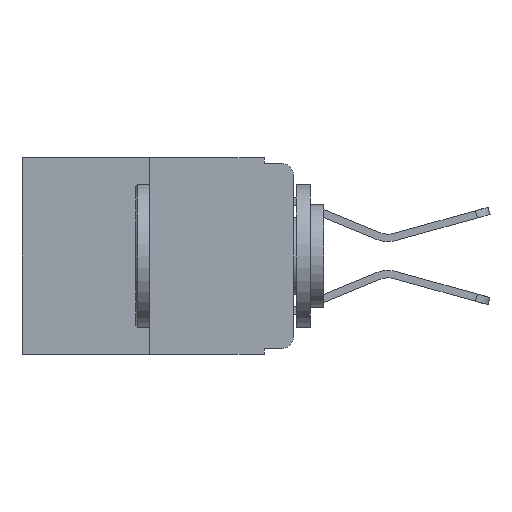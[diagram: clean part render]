
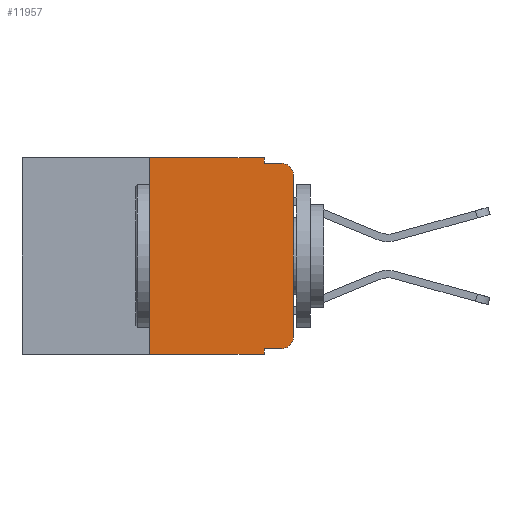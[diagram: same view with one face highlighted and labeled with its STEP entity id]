
A CAD part, left-side view. The second image highlights one B-rep face of the part: STEP entity #11957.
In plain terms, the highlighted planar face has unit normal (-1, 0, 0).
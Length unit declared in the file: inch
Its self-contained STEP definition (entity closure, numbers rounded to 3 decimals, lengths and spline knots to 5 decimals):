
#31 = CARTESIAN_POINT ( 'NONE',  ( 0., 0.051, 0. ) ) ;
#358 = DIRECTION ( 'NONE',  ( 0., 0., 1. ) ) ;
#479 = EDGE_CURVE ( 'NONE', #14245, #7207, #16732, .T. ) ;
#652 = CARTESIAN_POINT ( 'NONE',  ( 0., 0.473, 0. ) ) ;
#1036 = ORIENTED_EDGE ( 'NONE', *, *, #11001, .T. ) ;
#1067 = LINE ( 'NONE', #2929, #14947 ) ;
#1095 = VECTOR ( 'NONE', #3181, 39.37008 ) ;
#1126 = CARTESIAN_POINT ( 'NONE',  ( 0., 0.051, -0.333 ) ) ;
#1220 = DIRECTION ( 'NONE',  ( 0., 0., -1. ) ) ;
#1286 = EDGE_LOOP ( 'NONE', ( #9746, #17314, #14010, #10671, #15357, #8605, #1036, #13803, #14246, #10911 ) ) ;
#1747 = EDGE_CURVE ( 'NONE', #14640, #16593, #3908, .T. ) ;
#1892 = DIRECTION ( 'NONE',  ( 0., -1., 0. ) ) ;
#2015 = VECTOR ( 'NONE', #358, 39.37008 ) ;
#2631 = DIRECTION ( 'NONE',  ( 0., -1., 0. ) ) ;
#2929 = CARTESIAN_POINT ( 'NONE',  ( 0., 0.051, -0.01 ) ) ;
#3027 = CARTESIAN_POINT ( 'NONE',  ( 0., 0.02, -0.03 ) ) ;
#3181 = DIRECTION ( 'NONE',  ( 0., 0., -1. ) ) ;
#3718 = PLANE ( 'NONE',  #17920 ) ;
#3908 = LINE ( 'NONE', #16813, #15165 ) ;
#4431 = AXIS2_PLACEMENT_3D ( 'NONE', #6368, #7781, #1220 ) ;
#4578 = DIRECTION ( 'NONE',  ( 0., 0., -1. ) ) ;
#4724 = DIRECTION ( 'NONE',  ( 0., 0., 1. ) ) ;
#5534 = CARTESIAN_POINT ( 'NONE',  ( 0., 0.25, -0.343 ) ) ;
#5562 = LINE ( 'NONE', #1126, #12901 ) ;
#5783 = EDGE_CURVE ( 'NONE', #16965, #6079, #6066, .T. ) ;
#5942 = EDGE_CURVE ( 'NONE', #7207, #9414, #1067, .T. ) ;
#5958 = CARTESIAN_POINT ( 'NONE',  ( 0., 0.473, 0. ) ) ;
#6066 = LINE ( 'NONE', #7403, #2015 ) ;
#6079 = VERTEX_POINT ( 'NONE', #11698 ) ;
#6361 = CARTESIAN_POINT ( 'NONE',  ( 0., 0.473, -0.343 ) ) ;
#6368 = CARTESIAN_POINT ( 'NONE',  ( 0., 0.02, -0.313 ) ) ;
#6431 = VECTOR ( 'NONE', #4724, 39.37008 ) ;
#6530 = CARTESIAN_POINT ( 'NONE',  ( 0., 0., -0.313 ) ) ;
#6868 = VERTEX_POINT ( 'NONE', #5534 ) ;
#7207 = VERTEX_POINT ( 'NONE', #18071 ) ;
#7281 = CARTESIAN_POINT ( 'NONE',  ( 0., 0.25, 0. ) ) ;
#7403 = CARTESIAN_POINT ( 'NONE',  ( 0., 0., 0. ) ) ;
#7781 = DIRECTION ( 'NONE',  ( -1., 0., 0. ) ) ;
#8085 = EDGE_CURVE ( 'NONE', #10809, #16965, #10644, .T. ) ;
#8239 = DIRECTION ( 'NONE',  ( 1., 0., 0. ) ) ;
#8298 = VECTOR ( 'NONE', #9021, 39.37008 ) ;
#8605 = ORIENTED_EDGE ( 'NONE', *, *, #9204, .F. ) ;
#9021 = DIRECTION ( 'NONE',  ( 0., -1., 0. ) ) ;
#9089 = EDGE_CURVE ( 'NONE', #9663, #14245, #13051, .T. ) ;
#9204 = EDGE_CURVE ( 'NONE', #6868, #9663, #10361, .T. ) ;
#9414 = VERTEX_POINT ( 'NONE', #12554 ) ;
#9663 = VERTEX_POINT ( 'NONE', #7281 ) ;
#9746 = ORIENTED_EDGE ( 'NONE', *, *, #5783, .T. ) ;
#9839 = LINE ( 'NONE', #6361, #16976 ) ;
#10361 = LINE ( 'NONE', #14943, #6431 ) ;
#10479 = CARTESIAN_POINT ( 'NONE',  ( 0., 0.051, -0.343 ) ) ;
#10644 = CIRCLE ( 'NONE', #4431, 0.02 ) ;
#10671 = ORIENTED_EDGE ( 'NONE', *, *, #479, .F. ) ;
#10809 = VERTEX_POINT ( 'NONE', #15986 ) ;
#10911 = ORIENTED_EDGE ( 'NONE', *, *, #8085, .T. ) ;
#11001 = EDGE_CURVE ( 'NONE', #6868, #16593, #9839, .T. ) ;
#11698 = CARTESIAN_POINT ( 'NONE',  ( 0., 0., -0.03 ) ) ;
#11957 = ADVANCED_FACE ( 'NONE', ( #13862 ), #3718, .F. ) ;
#12554 = CARTESIAN_POINT ( 'NONE',  ( 0., 0.02, -0.01 ) ) ;
#12901 = VECTOR ( 'NONE', #2631, 39.37008 ) ;
#12910 = CARTESIAN_POINT ( 'NONE',  ( 0., 0.051, -0.333 ) ) ;
#13051 = LINE ( 'NONE', #5958, #8298 ) ;
#13290 = EDGE_CURVE ( 'NONE', #14640, #10809, #5562, .T. ) ;
#13358 = DIRECTION ( 'NONE',  ( -1., 0., 0. ) ) ;
#13624 = DIRECTION ( 'NONE',  ( 0., -1., 0. ) ) ;
#13803 = ORIENTED_EDGE ( 'NONE', *, *, #1747, .F. ) ;
#13862 = FACE_OUTER_BOUND ( 'NONE', #1286, .T. ) ;
#14010 = ORIENTED_EDGE ( 'NONE', *, *, #5942, .F. ) ;
#14171 = AXIS2_PLACEMENT_3D ( 'NONE', #3027, #13358, #4578 ) ;
#14229 = EDGE_CURVE ( 'NONE', #6079, #9414, #15763, .T. ) ;
#14245 = VERTEX_POINT ( 'NONE', #31 ) ;
#14246 = ORIENTED_EDGE ( 'NONE', *, *, #13290, .T. ) ;
#14640 = VERTEX_POINT ( 'NONE', #12910 ) ;
#14943 = CARTESIAN_POINT ( 'NONE',  ( 0., 0.25, 0. ) ) ;
#14947 = VECTOR ( 'NONE', #1892, 39.37008 ) ;
#15165 = VECTOR ( 'NONE', #17345, 39.37008 ) ;
#15357 = ORIENTED_EDGE ( 'NONE', *, *, #9089, .F. ) ;
#15763 = CIRCLE ( 'NONE', #14171, 0.02 ) ;
#15986 = CARTESIAN_POINT ( 'NONE',  ( 0., 0.02, -0.333 ) ) ;
#16576 = CARTESIAN_POINT ( 'NONE',  ( 0., 0.051, 0. ) ) ;
#16593 = VERTEX_POINT ( 'NONE', #10479 ) ;
#16732 = LINE ( 'NONE', #16576, #1095 ) ;
#16813 = CARTESIAN_POINT ( 'NONE',  ( 0., 0.051, 0. ) ) ;
#16965 = VERTEX_POINT ( 'NONE', #6530 ) ;
#16976 = VECTOR ( 'NONE', #13624, 39.37008 ) ;
#17314 = ORIENTED_EDGE ( 'NONE', *, *, #14229, .T. ) ;
#17345 = DIRECTION ( 'NONE',  ( 0., 0., -1. ) ) ;
#17920 = AXIS2_PLACEMENT_3D ( 'NONE', #652, #8239, #18241 ) ;
#18071 = CARTESIAN_POINT ( 'NONE',  ( 0., 0.051, -0.01 ) ) ;
#18241 = DIRECTION ( 'NONE',  ( 0., 0., -1. ) ) ;
